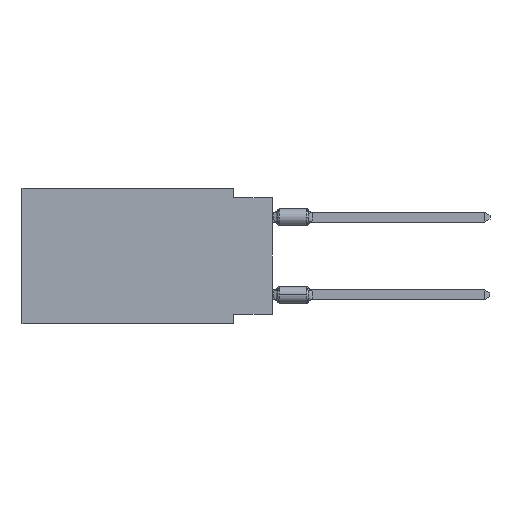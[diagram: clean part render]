
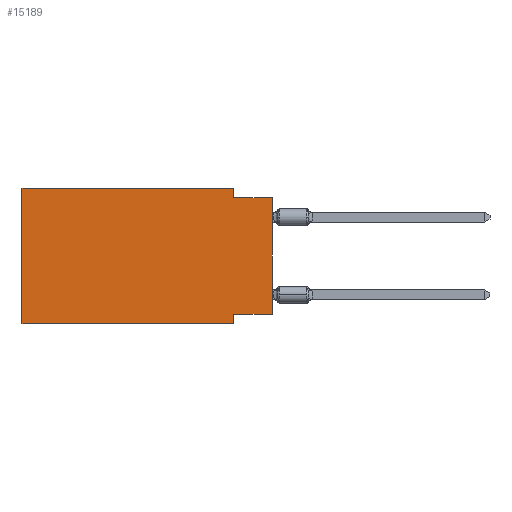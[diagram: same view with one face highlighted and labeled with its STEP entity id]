
A CAD part, left-side view. The second image highlights one B-rep face of the part: STEP entity #15189.
In plain terms, the highlighted planar face has unit normal (-1, 0, 0).
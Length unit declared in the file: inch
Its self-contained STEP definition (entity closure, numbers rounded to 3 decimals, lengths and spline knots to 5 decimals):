
#310 = DIRECTION ( 'NONE',  ( 0., 0., 1. ) ) ;
#349 = EDGE_CURVE ( 'NONE', #7445, #16306, #420, .T. ) ;
#420 = LINE ( 'NONE', #6829, #16746 ) ;
#1745 = CARTESIAN_POINT ( 'NONE',  ( 0., 0., -0.325 ) ) ;
#2268 = ORIENTED_EDGE ( 'NONE', *, *, #6368, .F. ) ;
#4513 = LINE ( 'NONE', #27733, #20670 ) ;
#4720 = ORIENTED_EDGE ( 'NONE', *, *, #349, .T. ) ;
#4809 = VECTOR ( 'NONE', #6937, 39.37008 ) ;
#4822 = ORIENTED_EDGE ( 'NONE', *, *, #15456, .F. ) ;
#4979 = VERTEX_POINT ( 'NONE', #26058 ) ;
#4996 = CARTESIAN_POINT ( 'NONE',  ( 0., 0., -0.025 ) ) ;
#5195 = CARTESIAN_POINT ( 'NONE',  ( 0., 0.645, 0. ) ) ;
#5266 = AXIS2_PLACEMENT_3D ( 'NONE', #18460, #6977, #9512 ) ;
#6368 = EDGE_CURVE ( 'NONE', #15852, #8199, #26789, .T. ) ;
#6829 = CARTESIAN_POINT ( 'NONE',  ( 0., 0.645, -0.35 ) ) ;
#6937 = DIRECTION ( 'NONE',  ( 0., -1., 0. ) ) ;
#6977 = DIRECTION ( 'NONE',  ( 1., 0., 0. ) ) ;
#7014 = VECTOR ( 'NONE', #310, 39.37008 ) ;
#7269 = EDGE_CURVE ( 'NONE', #10415, #4979, #4513, .T. ) ;
#7445 = VERTEX_POINT ( 'NONE', #14910 ) ;
#7665 = VECTOR ( 'NONE', #21971, 39.37008 ) ;
#8199 = VERTEX_POINT ( 'NONE', #26441 ) ;
#9059 = DIRECTION ( 'NONE',  ( 0., 0., -1. ) ) ;
#9512 = DIRECTION ( 'NONE',  ( 0., 0., -1. ) ) ;
#10165 = VERTEX_POINT ( 'NONE', #28595 ) ;
#10323 = ORIENTED_EDGE ( 'NONE', *, *, #21815, .F. ) ;
#10415 = VERTEX_POINT ( 'NONE', #16829 ) ;
#11578 = DIRECTION ( 'NONE',  ( 0., 0., -1. ) ) ;
#11613 = CARTESIAN_POINT ( 'NONE',  ( 0., 0.645, 0. ) ) ;
#11884 = FACE_OUTER_BOUND ( 'NONE', #22163, .T. ) ;
#12417 = CARTESIAN_POINT ( 'NONE',  ( 0., 0.1, -0.35 ) ) ;
#13269 = CARTESIAN_POINT ( 'NONE',  ( 0., 0.1, 0. ) ) ;
#13582 = DIRECTION ( 'NONE',  ( 0., 0., 1. ) ) ;
#13621 = LINE ( 'NONE', #4996, #4809 ) ;
#14910 = CARTESIAN_POINT ( 'NONE',  ( 0., 0.645, -0.35 ) ) ;
#15189 = ADVANCED_FACE ( 'NONE', ( #11884 ), #27369, .F. ) ;
#15456 = EDGE_CURVE ( 'NONE', #10415, #10165, #20209, .T. ) ;
#15677 = EDGE_CURVE ( 'NONE', #8199, #4979, #13621, .T. ) ;
#15793 = VECTOR ( 'NONE', #23288, 39.37008 ) ;
#15852 = VERTEX_POINT ( 'NONE', #13269 ) ;
#15982 = CARTESIAN_POINT ( 'NONE',  ( 0., 0.1, -0.35 ) ) ;
#16028 = EDGE_CURVE ( 'NONE', #19498, #15852, #21201, .T. ) ;
#16306 = VERTEX_POINT ( 'NONE', #15982 ) ;
#16746 = VECTOR ( 'NONE', #24990, 39.37008 ) ;
#16829 = CARTESIAN_POINT ( 'NONE',  ( 0., 0., -0.325 ) ) ;
#16903 = CARTESIAN_POINT ( 'NONE',  ( 0., 0.645, 0. ) ) ;
#18172 = LINE ( 'NONE', #12417, #23596 ) ;
#18460 = CARTESIAN_POINT ( 'NONE',  ( 0., 0.645, 0. ) ) ;
#19498 = VERTEX_POINT ( 'NONE', #5195 ) ;
#20209 = LINE ( 'NONE', #1745, #7665 ) ;
#20605 = ORIENTED_EDGE ( 'NONE', *, *, #15677, .F. ) ;
#20670 = VECTOR ( 'NONE', #13582, 39.37008 ) ;
#20855 = EDGE_CURVE ( 'NONE', #10165, #16306, #18172, .T. ) ;
#21097 = VECTOR ( 'NONE', #9059, 39.37008 ) ;
#21201 = LINE ( 'NONE', #16903, #15793 ) ;
#21815 = EDGE_CURVE ( 'NONE', #7445, #19498, #25175, .T. ) ;
#21971 = DIRECTION ( 'NONE',  ( 0., 1., 0. ) ) ;
#22163 = EDGE_LOOP ( 'NONE', ( #25993, #20605, #2268, #25669, #10323, #4720, #23658, #4822 ) ) ;
#22309 = CARTESIAN_POINT ( 'NONE',  ( 0., 0.1, 0. ) ) ;
#23288 = DIRECTION ( 'NONE',  ( 0., -1., 0. ) ) ;
#23596 = VECTOR ( 'NONE', #11578, 39.37008 ) ;
#23658 = ORIENTED_EDGE ( 'NONE', *, *, #20855, .F. ) ;
#24990 = DIRECTION ( 'NONE',  ( 0., -1., 0. ) ) ;
#25175 = LINE ( 'NONE', #11613, #7014 ) ;
#25669 = ORIENTED_EDGE ( 'NONE', *, *, #16028, .F. ) ;
#25993 = ORIENTED_EDGE ( 'NONE', *, *, #7269, .T. ) ;
#26058 = CARTESIAN_POINT ( 'NONE',  ( 0., 0., -0.025 ) ) ;
#26441 = CARTESIAN_POINT ( 'NONE',  ( 0., 0.1, -0.025 ) ) ;
#26789 = LINE ( 'NONE', #22309, #21097 ) ;
#27369 = PLANE ( 'NONE',  #5266 ) ;
#27733 = CARTESIAN_POINT ( 'NONE',  ( 0., 0., 0. ) ) ;
#28595 = CARTESIAN_POINT ( 'NONE',  ( 0., 0.1, -0.325 ) ) ;
